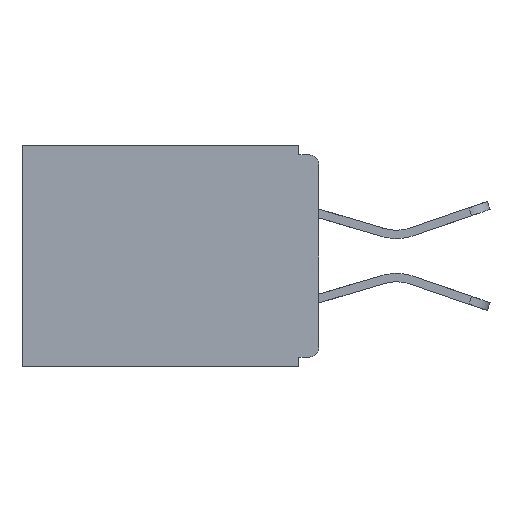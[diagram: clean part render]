
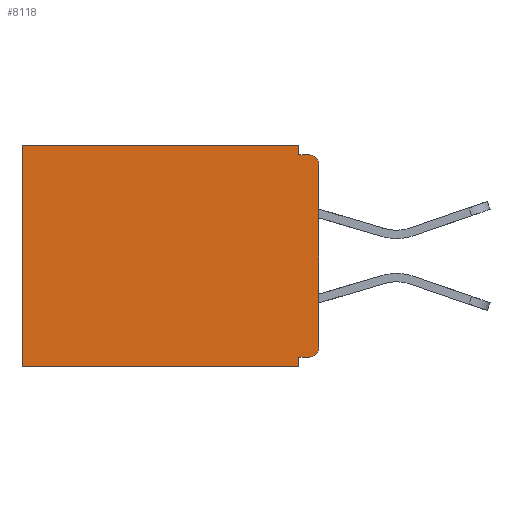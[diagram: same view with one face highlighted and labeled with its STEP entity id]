
A CAD part, left-side view. The second image highlights one B-rep face of the part: STEP entity #8118.
In plain terms, the highlighted planar face has unit normal (-1, 0, 0).
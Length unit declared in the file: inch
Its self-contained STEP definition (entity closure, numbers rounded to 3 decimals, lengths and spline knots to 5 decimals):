
#467 = ORIENTED_EDGE ( 'NONE', *, *, #6868, .T. ) ;
#1126 = CARTESIAN_POINT ( 'NONE',  ( 0.298, 0., -0.313 ) ) ;
#1353 = VECTOR ( 'NONE', #3537, 39.37008 ) ;
#1530 = DIRECTION ( 'NONE',  ( 0., 0., -1. ) ) ;
#1603 = CARTESIAN_POINT ( 'NONE',  ( 0.298, 0.46, 0. ) ) ;
#1766 = DIRECTION ( 'NONE',  ( 0., 1., 0. ) ) ;
#1929 = EDGE_CURVE ( 'NONE', #4950, #19668, #6454, .T. ) ;
#2274 = LINE ( 'NONE', #22182, #11062 ) ;
#2590 = CARTESIAN_POINT ( 'NONE',  ( 0.298, 0.46, -0.343 ) ) ;
#2632 = VERTEX_POINT ( 'NONE', #3673 ) ;
#2692 = LINE ( 'NONE', #7169, #13955 ) ;
#3380 = CARTESIAN_POINT ( 'NONE',  ( 0.298, 0.031, -0.015 ) ) ;
#3537 = DIRECTION ( 'NONE',  ( 0., 1., 0. ) ) ;
#3639 = CARTESIAN_POINT ( 'NONE',  ( 0.298, 0., 0. ) ) ;
#3673 = CARTESIAN_POINT ( 'NONE',  ( 0.298, 0.031, -0.343 ) ) ;
#3735 = AXIS2_PLACEMENT_3D ( 'NONE', #15649, #5228, #17343 ) ;
#3783 = ORIENTED_EDGE ( 'NONE', *, *, #15272, .F. ) ;
#4052 = DIRECTION ( 'NONE',  ( 0., 0., -1. ) ) ;
#4324 = LINE ( 'NONE', #1603, #12329 ) ;
#4559 = FACE_OUTER_BOUND ( 'NONE', #14436, .T. ) ;
#4618 = CARTESIAN_POINT ( 'NONE',  ( 0.298, 0.031, -0.343 ) ) ;
#4673 = LINE ( 'NONE', #4618, #7719 ) ;
#4700 = VERTEX_POINT ( 'NONE', #20850 ) ;
#4749 = ORIENTED_EDGE ( 'NONE', *, *, #1929, .T. ) ;
#4950 = VERTEX_POINT ( 'NONE', #9170 ) ;
#5016 = PLANE ( 'NONE',  #11945 ) ;
#5139 = ORIENTED_EDGE ( 'NONE', *, *, #17783, .T. ) ;
#5228 = DIRECTION ( 'NONE',  ( -1., 0., 0. ) ) ;
#5382 = DIRECTION ( 'NONE',  ( 0., 1., 0. ) ) ;
#5734 = VERTEX_POINT ( 'NONE', #3380 ) ;
#6033 = LINE ( 'NONE', #18899, #1353 ) ;
#6253 = VERTEX_POINT ( 'NONE', #8325 ) ;
#6260 = EDGE_CURVE ( 'NONE', #4700, #2632, #4673, .T. ) ;
#6454 = CIRCLE ( 'NONE', #3735, 0.015 ) ;
#6868 = EDGE_CURVE ( 'NONE', #13900, #6253, #6033, .T. ) ;
#7169 = CARTESIAN_POINT ( 'NONE',  ( 0.298, 0., -0.328 ) ) ;
#7329 = EDGE_CURVE ( 'NONE', #2632, #19558, #8211, .T. ) ;
#7719 = VECTOR ( 'NONE', #14988, 39.37008 ) ;
#7889 = LINE ( 'NONE', #12999, #18302 ) ;
#8118 = ADVANCED_FACE ( 'NONE', ( #4559 ), #5016, .F. ) ;
#8211 = LINE ( 'NONE', #21098, #21349 ) ;
#8316 = DIRECTION ( 'NONE',  ( 0., 0., -1. ) ) ;
#8325 = CARTESIAN_POINT ( 'NONE',  ( 0.298, 0.46, 0. ) ) ;
#8805 = LINE ( 'NONE', #3639, #12112 ) ;
#9033 = VERTEX_POINT ( 'NONE', #17015 ) ;
#9170 = CARTESIAN_POINT ( 'NONE',  ( 0.298, 0.015, -0.328 ) ) ;
#9225 = DIRECTION ( 'NONE',  ( 0., 0., -1. ) ) ;
#9282 = DIRECTION ( 'NONE',  ( -1., 0., 0. ) ) ;
#11062 = VECTOR ( 'NONE', #17498, 39.37008 ) ;
#11662 = AXIS2_PLACEMENT_3D ( 'NONE', #12748, #9282, #4052 ) ;
#11945 = AXIS2_PLACEMENT_3D ( 'NONE', #18813, #17351, #8316 ) ;
#12034 = VERTEX_POINT ( 'NONE', #17582 ) ;
#12112 = VECTOR ( 'NONE', #17888, 39.37008 ) ;
#12119 = EDGE_CURVE ( 'NONE', #9033, #12034, #12980, .T. ) ;
#12329 = VECTOR ( 'NONE', #1530, 39.37008 ) ;
#12748 = CARTESIAN_POINT ( 'NONE',  ( 0.298, 0.015, -0.03 ) ) ;
#12791 = EDGE_CURVE ( 'NONE', #5734, #12034, #2274, .T. ) ;
#12980 = CIRCLE ( 'NONE', #11662, 0.015 ) ;
#12999 = CARTESIAN_POINT ( 'NONE',  ( 0.298, 0.031, -0.343 ) ) ;
#13900 = VERTEX_POINT ( 'NONE', #18011 ) ;
#13955 = VECTOR ( 'NONE', #1766, 39.37008 ) ;
#14436 = EDGE_LOOP ( 'NONE', ( #16899, #22187, #18922, #467, #5139, #19389, #15847, #3783, #4749, #15006 ) ) ;
#14988 = DIRECTION ( 'NONE',  ( 0., 0., -1. ) ) ;
#15006 = ORIENTED_EDGE ( 'NONE', *, *, #16688, .F. ) ;
#15272 = EDGE_CURVE ( 'NONE', #4950, #4700, #2692, .T. ) ;
#15649 = CARTESIAN_POINT ( 'NONE',  ( 0.298, 0.015, -0.313 ) ) ;
#15847 = ORIENTED_EDGE ( 'NONE', *, *, #6260, .F. ) ;
#15869 = EDGE_CURVE ( 'NONE', #13900, #5734, #7889, .T. ) ;
#16688 = EDGE_CURVE ( 'NONE', #9033, #19668, #8805, .T. ) ;
#16899 = ORIENTED_EDGE ( 'NONE', *, *, #12119, .T. ) ;
#17015 = CARTESIAN_POINT ( 'NONE',  ( 0.298, 0., -0.03 ) ) ;
#17343 = DIRECTION ( 'NONE',  ( 0., 0., -1. ) ) ;
#17351 = DIRECTION ( 'NONE',  ( 1., 0., 0. ) ) ;
#17498 = DIRECTION ( 'NONE',  ( 0., -1., 0. ) ) ;
#17582 = CARTESIAN_POINT ( 'NONE',  ( 0.298, 0.015, -0.015 ) ) ;
#17783 = EDGE_CURVE ( 'NONE', #6253, #19558, #4324, .T. ) ;
#17888 = DIRECTION ( 'NONE',  ( 0., 0., -1. ) ) ;
#18011 = CARTESIAN_POINT ( 'NONE',  ( 0.298, 0.031, 0. ) ) ;
#18302 = VECTOR ( 'NONE', #9225, 39.37008 ) ;
#18813 = CARTESIAN_POINT ( 'NONE',  ( 0.298, 0., 0. ) ) ;
#18899 = CARTESIAN_POINT ( 'NONE',  ( 0.298, 0., 0. ) ) ;
#18922 = ORIENTED_EDGE ( 'NONE', *, *, #15869, .F. ) ;
#19389 = ORIENTED_EDGE ( 'NONE', *, *, #7329, .F. ) ;
#19558 = VERTEX_POINT ( 'NONE', #2590 ) ;
#19668 = VERTEX_POINT ( 'NONE', #1126 ) ;
#20850 = CARTESIAN_POINT ( 'NONE',  ( 0.298, 0.031, -0.328 ) ) ;
#21098 = CARTESIAN_POINT ( 'NONE',  ( 0.298, 0., -0.343 ) ) ;
#21349 = VECTOR ( 'NONE', #5382, 39.37008 ) ;
#22182 = CARTESIAN_POINT ( 'NONE',  ( 0.298, 0., -0.015 ) ) ;
#22187 = ORIENTED_EDGE ( 'NONE', *, *, #12791, .F. ) ;
